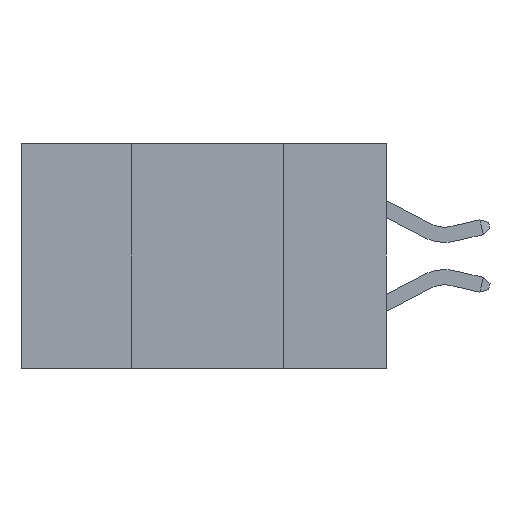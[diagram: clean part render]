
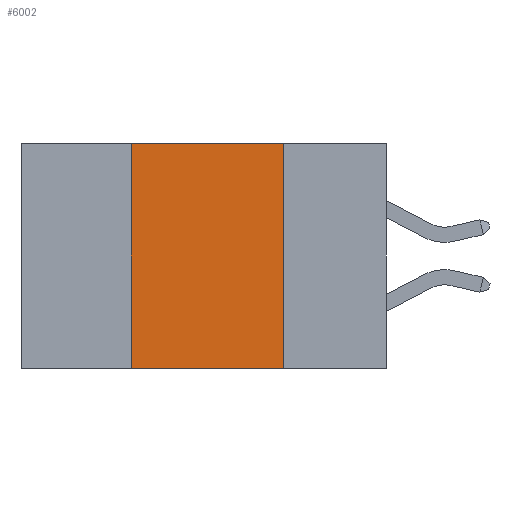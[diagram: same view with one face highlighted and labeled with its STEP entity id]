
A CAD part, left-side view. The second image highlights one B-rep face of the part: STEP entity #6002.
In plain terms, the highlighted planar face has unit normal (-1, 0, 0).
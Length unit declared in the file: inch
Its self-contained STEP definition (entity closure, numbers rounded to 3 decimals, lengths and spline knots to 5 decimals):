
#187 = ORIENTED_EDGE ( 'NONE', *, *, #370, .F. ) ;
#370 = EDGE_CURVE ( 'NONE', #9685, #8219, #5006, .T. ) ;
#2618 = AXIS2_PLACEMENT_3D ( 'NONE', #9030, #9010, #8995 ) ;
#4578 = VECTOR ( 'NONE', #13791, 39.37008 ) ;
#4608 = EDGE_LOOP ( 'NONE', ( #9828, #14989, #187, #16140 ) ) ;
#4950 = EDGE_CURVE ( 'NONE', #6503, #7742, #7660, .T. ) ;
#5006 = LINE ( 'NONE', #13841, #4578 ) ;
#5133 = LINE ( 'NONE', #14490, #15388 ) ;
#5227 = CARTESIAN_POINT ( 'NONE',  ( 0., 0.17, 0. ) ) ;
#5565 = CARTESIAN_POINT ( 'NONE',  ( 0., 0.17, -0.37 ) ) ;
#6002 = ADVANCED_FACE ( 'NONE', ( #15300 ), #9186, .F. ) ;
#6503 = VERTEX_POINT ( 'NONE', #5227 ) ;
#6628 = LINE ( 'NONE', #13886, #10214 ) ;
#7660 = LINE ( 'NONE', #17181, #13927 ) ;
#7742 = VERTEX_POINT ( 'NONE', #5565 ) ;
#8219 = VERTEX_POINT ( 'NONE', #10313 ) ;
#8995 = DIRECTION ( 'NONE',  ( 0., 0., -1. ) ) ;
#9010 = DIRECTION ( 'NONE',  ( 1., 0., 0. ) ) ;
#9014 = EDGE_CURVE ( 'NONE', #9685, #7742, #6628, .T. ) ;
#9030 = CARTESIAN_POINT ( 'NONE',  ( 0., 0.6, 0. ) ) ;
#9186 = PLANE ( 'NONE',  #2618 ) ;
#9685 = VERTEX_POINT ( 'NONE', #16192 ) ;
#9828 = ORIENTED_EDGE ( 'NONE', *, *, #4950, .F. ) ;
#10214 = VECTOR ( 'NONE', #14087, 39.37008 ) ;
#10313 = CARTESIAN_POINT ( 'NONE',  ( 0., 0.42, 0. ) ) ;
#13791 = DIRECTION ( 'NONE',  ( 0., 0., 1. ) ) ;
#13841 = CARTESIAN_POINT ( 'NONE',  ( 0., 0.42, -0.37 ) ) ;
#13886 = CARTESIAN_POINT ( 'NONE',  ( 0., 0.6, -0.37 ) ) ;
#13927 = VECTOR ( 'NONE', #17168, 39.37008 ) ;
#14087 = DIRECTION ( 'NONE',  ( 0., -1., 0. ) ) ;
#14490 = CARTESIAN_POINT ( 'NONE',  ( 0., 0.6, 0. ) ) ;
#14989 = ORIENTED_EDGE ( 'NONE', *, *, #15434, .F. ) ;
#15300 = FACE_OUTER_BOUND ( 'NONE', #4608, .T. ) ;
#15388 = VECTOR ( 'NONE', #16988, 39.37008 ) ;
#15434 = EDGE_CURVE ( 'NONE', #8219, #6503, #5133, .T. ) ;
#16140 = ORIENTED_EDGE ( 'NONE', *, *, #9014, .T. ) ;
#16192 = CARTESIAN_POINT ( 'NONE',  ( 0., 0.42, -0.37 ) ) ;
#16988 = DIRECTION ( 'NONE',  ( 0., -1., 0. ) ) ;
#17168 = DIRECTION ( 'NONE',  ( 0., 0., -1. ) ) ;
#17181 = CARTESIAN_POINT ( 'NONE',  ( 0., 0.17, -0.37 ) ) ;
